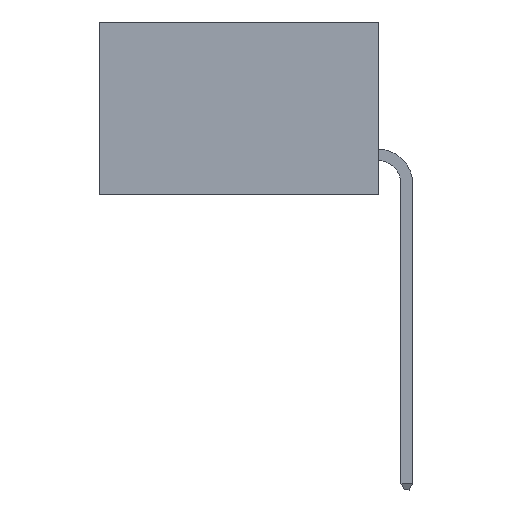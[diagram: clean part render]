
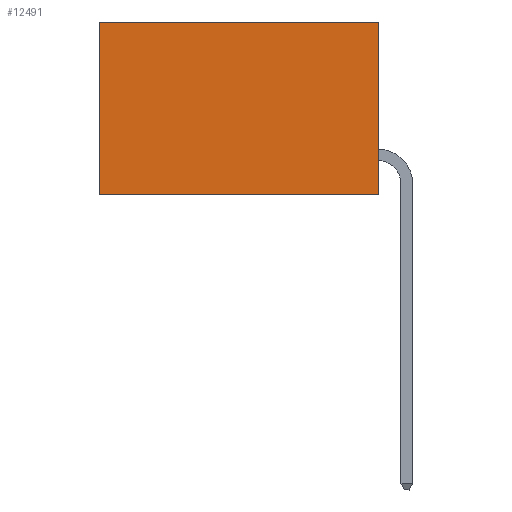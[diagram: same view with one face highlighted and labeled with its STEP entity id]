
A CAD part, left-side view. The second image highlights one B-rep face of the part: STEP entity #12491.
In plain terms, the highlighted planar face has unit normal (-1, 0, 0).
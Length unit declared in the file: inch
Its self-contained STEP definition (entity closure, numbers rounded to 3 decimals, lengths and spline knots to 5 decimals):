
#1487 = CARTESIAN_POINT ( 'NONE',  ( 0.2615, 0.6, 0. ) ) ;
#3175 = LINE ( 'NONE', #24582, #20998 ) ;
#4059 = CARTESIAN_POINT ( 'NONE',  ( 0.2615, 0., -0.37 ) ) ;
#4197 = DIRECTION ( 'NONE',  ( 0., 0., -1. ) ) ;
#7477 = LINE ( 'NONE', #13828, #25163 ) ;
#7724 = DIRECTION ( 'NONE',  ( 0., 0., -1. ) ) ;
#8526 = ORIENTED_EDGE ( 'NONE', *, *, #25148, .F. ) ;
#8656 = VERTEX_POINT ( 'NONE', #1487 ) ;
#9749 = DIRECTION ( 'NONE',  ( 1., 0., 0. ) ) ;
#11172 = DIRECTION ( 'NONE',  ( 0., 0., -1. ) ) ;
#11232 = EDGE_LOOP ( 'NONE', ( #18910, #8526, #19935, #11899 ) ) ;
#11899 = ORIENTED_EDGE ( 'NONE', *, *, #23117, .T. ) ;
#12037 = CARTESIAN_POINT ( 'NONE',  ( 0.2615, 0., -0.37 ) ) ;
#12356 = CARTESIAN_POINT ( 'NONE',  ( 0.2615, 0., -0.37 ) ) ;
#12491 = ADVANCED_FACE ( 'NONE', ( #13971 ), #15506, .F. ) ;
#12956 = DIRECTION ( 'NONE',  ( 0., 1., 0. ) ) ;
#13828 = CARTESIAN_POINT ( 'NONE',  ( 0.2615, 0.6, -0.37 ) ) ;
#13971 = FACE_OUTER_BOUND ( 'NONE', #11232, .T. ) ;
#14749 = LINE ( 'NONE', #20952, #24669 ) ;
#15018 = DIRECTION ( 'NONE',  ( 0., 1., 0. ) ) ;
#15389 = AXIS2_PLACEMENT_3D ( 'NONE', #12037, #9749, #4197 ) ;
#15506 = PLANE ( 'NONE',  #15389 ) ;
#16341 = CARTESIAN_POINT ( 'NONE',  ( 0.2615, 0., 0. ) ) ;
#18566 = EDGE_CURVE ( 'NONE', #18875, #23353, #14749, .T. ) ;
#18875 = VERTEX_POINT ( 'NONE', #16341 ) ;
#18910 = ORIENTED_EDGE ( 'NONE', *, *, #22232, .T. ) ;
#19935 = ORIENTED_EDGE ( 'NONE', *, *, #18566, .F. ) ;
#20190 = LINE ( 'NONE', #12356, #21994 ) ;
#20952 = CARTESIAN_POINT ( 'NONE',  ( 0.2615, 0., -0.37 ) ) ;
#20998 = VECTOR ( 'NONE', #12956, 39.37008 ) ;
#21926 = CARTESIAN_POINT ( 'NONE',  ( 0.2615, 0.6, -0.37 ) ) ;
#21994 = VECTOR ( 'NONE', #15018, 39.37008 ) ;
#22232 = EDGE_CURVE ( 'NONE', #8656, #23426, #7477, .T. ) ;
#23117 = EDGE_CURVE ( 'NONE', #18875, #8656, #3175, .T. ) ;
#23353 = VERTEX_POINT ( 'NONE', #4059 ) ;
#23426 = VERTEX_POINT ( 'NONE', #21926 ) ;
#24582 = CARTESIAN_POINT ( 'NONE',  ( 0.2615, 0., 0. ) ) ;
#24669 = VECTOR ( 'NONE', #11172, 39.37008 ) ;
#25148 = EDGE_CURVE ( 'NONE', #23353, #23426, #20190, .T. ) ;
#25163 = VECTOR ( 'NONE', #7724, 39.37008 ) ;
